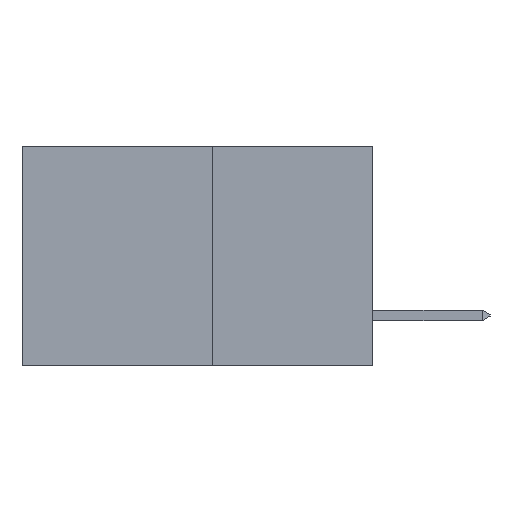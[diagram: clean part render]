
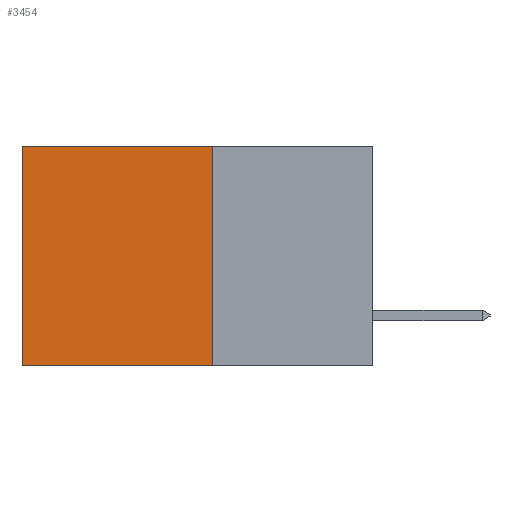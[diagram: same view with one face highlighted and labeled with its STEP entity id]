
A CAD part, left-side view. The second image highlights one B-rep face of the part: STEP entity #3454.
In plain terms, the highlighted planar face has unit normal (-1, 0, 0).
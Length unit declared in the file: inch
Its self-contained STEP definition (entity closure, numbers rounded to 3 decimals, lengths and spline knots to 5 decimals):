
#19 = ORIENTED_EDGE ( 'NONE', *, *, #14065, .T. ) ;
#782 = EDGE_LOOP ( 'NONE', ( #14300, #14336, #14475, #19 ) ) ;
#1286 = FACE_OUTER_BOUND ( 'NONE', #782, .T. ) ;
#1411 = VERTEX_POINT ( 'NONE', #7593 ) ;
#1429 = CARTESIAN_POINT ( 'NONE',  ( 0.277, 0.59, -0.37 ) ) ;
#2335 = PLANE ( 'NONE',  #9078 ) ;
#2758 = DIRECTION ( 'NONE',  ( 0., 0., -1. ) ) ;
#2918 = DIRECTION ( 'NONE',  ( 1., 0., 0. ) ) ;
#3284 = DIRECTION ( 'NONE',  ( 0., 0., -1. ) ) ;
#3454 = ADVANCED_FACE ( 'NONE', ( #1286 ), #2335, .F. ) ;
#3921 = LINE ( 'NONE', #20746, #7922 ) ;
#6109 = VECTOR ( 'NONE', #10390, 39.37008 ) ;
#6247 = VERTEX_POINT ( 'NONE', #19410 ) ;
#6533 = EDGE_CURVE ( 'NONE', #1411, #6247, #3921, .T. ) ;
#7593 = CARTESIAN_POINT ( 'NONE',  ( 0.277, 0.27, 0. ) ) ;
#7683 = VECTOR ( 'NONE', #19977, 39.37008 ) ;
#7872 = EDGE_CURVE ( 'NONE', #10577, #19123, #20874, .T. ) ;
#7922 = VECTOR ( 'NONE', #20235, 39.37008 ) ;
#7940 = EDGE_CURVE ( 'NONE', #6247, #19123, #19849, .T. ) ;
#8602 = CARTESIAN_POINT ( 'NONE',  ( 0.277, 0.27, -0.37 ) ) ;
#9078 = AXIS2_PLACEMENT_3D ( 'NONE', #14477, #2918, #2758 ) ;
#10390 = DIRECTION ( 'NONE',  ( 0., 1., 0. ) ) ;
#10577 = VERTEX_POINT ( 'NONE', #21757 ) ;
#11836 = VECTOR ( 'NONE', #3284, 39.37008 ) ;
#12928 = LINE ( 'NONE', #16572, #7683 ) ;
#14065 = EDGE_CURVE ( 'NONE', #1411, #10577, #12928, .T. ) ;
#14300 = ORIENTED_EDGE ( 'NONE', *, *, #7872, .T. ) ;
#14336 = ORIENTED_EDGE ( 'NONE', *, *, #7940, .F. ) ;
#14475 = ORIENTED_EDGE ( 'NONE', *, *, #6533, .F. ) ;
#14477 = CARTESIAN_POINT ( 'NONE',  ( 0.277, 0.27, -0.37 ) ) ;
#16572 = CARTESIAN_POINT ( 'NONE',  ( 0.277, 0.27, 0. ) ) ;
#18104 = CARTESIAN_POINT ( 'NONE',  ( 0.277, 0.59, -0.37 ) ) ;
#19123 = VERTEX_POINT ( 'NONE', #18104 ) ;
#19410 = CARTESIAN_POINT ( 'NONE',  ( 0.277, 0.27, -0.37 ) ) ;
#19849 = LINE ( 'NONE', #8602, #6109 ) ;
#19977 = DIRECTION ( 'NONE',  ( 0., 1., 0. ) ) ;
#20235 = DIRECTION ( 'NONE',  ( 0., 0., -1. ) ) ;
#20746 = CARTESIAN_POINT ( 'NONE',  ( 0.277, 0.27, -0.37 ) ) ;
#20874 = LINE ( 'NONE', #1429, #11836 ) ;
#21757 = CARTESIAN_POINT ( 'NONE',  ( 0.277, 0.59, 0. ) ) ;
